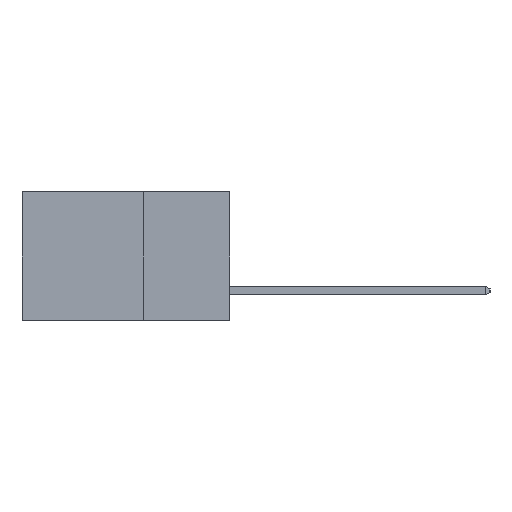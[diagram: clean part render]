
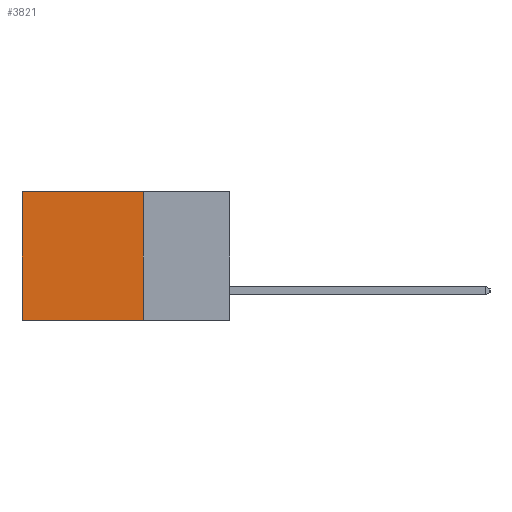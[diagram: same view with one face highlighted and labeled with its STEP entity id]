
A CAD part, left-side view. The second image highlights one B-rep face of the part: STEP entity #3821.
In plain terms, the highlighted planar face has unit normal (-1, 0, 0).
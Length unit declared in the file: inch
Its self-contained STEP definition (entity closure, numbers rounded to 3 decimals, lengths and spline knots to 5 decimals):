
#396 = LINE ( 'NONE', #6851, #25064 ) ;
#461 = DIRECTION ( 'NONE',  ( 0., 0., -1. ) ) ;
#486 = CARTESIAN_POINT ( 'NONE',  ( 0.2615, 0.6, 0. ) ) ;
#516 = CARTESIAN_POINT ( 'NONE',  ( 0.2615, 0.25, -0.37 ) ) ;
#1178 = VERTEX_POINT ( 'NONE', #23817 ) ;
#2143 = AXIS2_PLACEMENT_3D ( 'NONE', #14907, #14584, #14529 ) ;
#2508 = VERTEX_POINT ( 'NONE', #15900 ) ;
#2694 = VECTOR ( 'NONE', #23353, 39.37008 ) ;
#3467 = EDGE_CURVE ( 'NONE', #2508, #10070, #8590, .T. ) ;
#3621 = ORIENTED_EDGE ( 'NONE', *, *, #13837, .F. ) ;
#3821 = ADVANCED_FACE ( 'NONE', ( #20184 ), #14616, .F. ) ;
#4692 = EDGE_CURVE ( 'NONE', #10070, #1178, #396, .T. ) ;
#5992 = VECTOR ( 'NONE', #461, 39.37008 ) ;
#6692 = ORIENTED_EDGE ( 'NONE', *, *, #3467, .T. ) ;
#6851 = CARTESIAN_POINT ( 'NONE',  ( 0.2615, 0.6, -0.37 ) ) ;
#7286 = DIRECTION ( 'NONE',  ( 0., 0., -1. ) ) ;
#8590 = LINE ( 'NONE', #23334, #2694 ) ;
#9165 = DIRECTION ( 'NONE',  ( 0., 1., 0. ) ) ;
#9271 = CARTESIAN_POINT ( 'NONE',  ( 0.2615, 0.25, -0.37 ) ) ;
#10070 = VERTEX_POINT ( 'NONE', #486 ) ;
#11441 = EDGE_CURVE ( 'NONE', #15177, #1178, #13287, .T. ) ;
#12433 = ORIENTED_EDGE ( 'NONE', *, *, #4692, .T. ) ;
#12608 = EDGE_LOOP ( 'NONE', ( #12433, #17725, #3621, #6692 ) ) ;
#13287 = LINE ( 'NONE', #9271, #22933 ) ;
#13837 = EDGE_CURVE ( 'NONE', #2508, #15177, #21594, .T. ) ;
#14529 = DIRECTION ( 'NONE',  ( 0., 0., -1. ) ) ;
#14584 = DIRECTION ( 'NONE',  ( 1., 0., 0. ) ) ;
#14616 = PLANE ( 'NONE',  #2143 ) ;
#14907 = CARTESIAN_POINT ( 'NONE',  ( 0.2615, 0.25, -0.37 ) ) ;
#15177 = VERTEX_POINT ( 'NONE', #18585 ) ;
#15900 = CARTESIAN_POINT ( 'NONE',  ( 0.2615, 0.25, 0. ) ) ;
#17725 = ORIENTED_EDGE ( 'NONE', *, *, #11441, .F. ) ;
#18585 = CARTESIAN_POINT ( 'NONE',  ( 0.2615, 0.25, -0.37 ) ) ;
#20184 = FACE_OUTER_BOUND ( 'NONE', #12608, .T. ) ;
#21594 = LINE ( 'NONE', #516, #5992 ) ;
#22933 = VECTOR ( 'NONE', #9165, 39.37008 ) ;
#23334 = CARTESIAN_POINT ( 'NONE',  ( 0.2615, 0.25, 0. ) ) ;
#23353 = DIRECTION ( 'NONE',  ( 0., 1., 0. ) ) ;
#23817 = CARTESIAN_POINT ( 'NONE',  ( 0.2615, 0.6, -0.37 ) ) ;
#25064 = VECTOR ( 'NONE', #7286, 39.37008 ) ;
